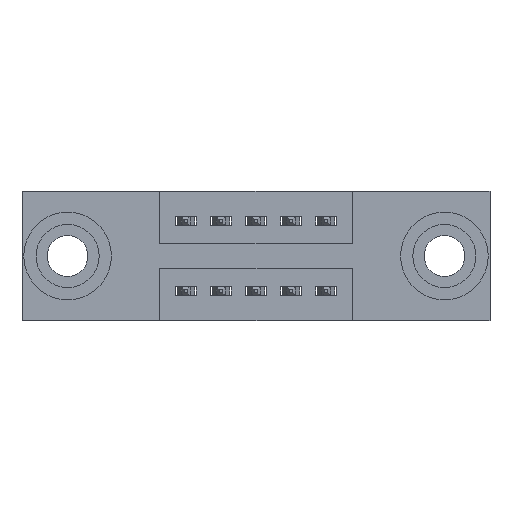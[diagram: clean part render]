
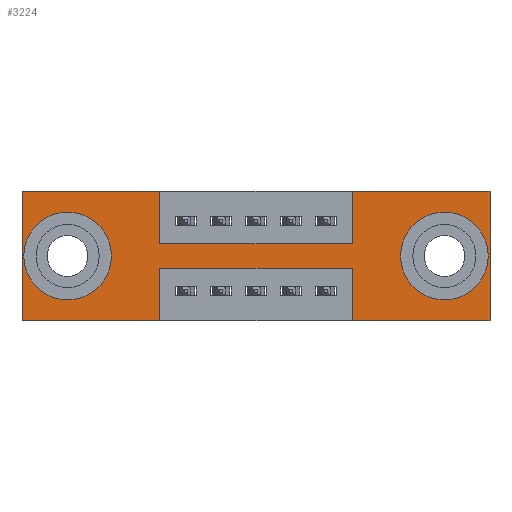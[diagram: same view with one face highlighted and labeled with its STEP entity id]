
A CAD part, front view. The second image highlights one B-rep face of the part: STEP entity #3224.
In plain terms, the highlighted planar face has unit normal (0, -1, 0).
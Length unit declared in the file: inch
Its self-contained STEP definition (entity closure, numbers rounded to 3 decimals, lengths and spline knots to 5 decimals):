
#199 = VERTEX_POINT ( 'NONE', #5408 ) ;
#202 = CARTESIAN_POINT ( 'NONE',  ( 0.9425, 0., -0.22 ) ) ;
#220 = VERTEX_POINT ( 'NONE', #5015 ) ;
#273 = LINE ( 'NONE', #3442, #8109 ) ;
#441 = CARTESIAN_POINT ( 'NONE',  ( 1.205, 0., -0.107 ) ) ;
#451 = EDGE_CURVE ( 'NONE', #7495, #7640, #5093, .T. ) ;
#491 = DIRECTION ( 'NONE',  ( 0., 1., 0. ) ) ;
#572 = AXIS2_PLACEMENT_3D ( 'NONE', #5320, #583, #6077 ) ;
#583 = DIRECTION ( 'NONE',  ( 0., 1., 0. ) ) ;
#598 = ORIENTED_EDGE ( 'NONE', *, *, #2854, .F. ) ;
#739 = VECTOR ( 'NONE', #2907, 39.37008 ) ;
#806 = EDGE_CURVE ( 'NONE', #3366, #220, #8985, .T. ) ;
#825 = VECTOR ( 'NONE', #2580, 39.37008 ) ;
#908 = VECTOR ( 'NONE', #1467, 39.37008 ) ;
#920 = EDGE_CURVE ( 'NONE', #6733, #3366, #6147, .T. ) ;
#1013 = ORIENTED_EDGE ( 'NONE', *, *, #6311, .F. ) ;
#1037 = VERTEX_POINT ( 'NONE', #5491 ) ;
#1129 = CARTESIAN_POINT ( 'NONE',  ( 0.9425, 0., 0. ) ) ;
#1196 = VERTEX_POINT ( 'NONE', #3708 ) ;
#1205 = VERTEX_POINT ( 'NONE', #3588 ) ;
#1379 = ORIENTED_EDGE ( 'NONE', *, *, #4823, .T. ) ;
#1417 = VECTOR ( 'NONE', #8301, 39.37008 ) ;
#1467 = DIRECTION ( 'NONE',  ( -1., 0., 0. ) ) ;
#1501 = FACE_OUTER_BOUND ( 'NONE', #8393, .T. ) ;
#1577 = CIRCLE ( 'NONE', #572, 0.078 ) ;
#1755 = CARTESIAN_POINT ( 'NONE',  ( 0., 0., 0. ) ) ;
#1802 = LINE ( 'NONE', #2672, #3683 ) ;
#1833 = DIRECTION ( 'NONE',  ( 0., 0., -1. ) ) ;
#1900 = ORIENTED_EDGE ( 'NONE', *, *, #8420, .F. ) ;
#1905 = CARTESIAN_POINT ( 'NONE',  ( 0.13, 0., -0.185 ) ) ;
#1915 = EDGE_LOOP ( 'NONE', ( #6055, #2595 ) ) ;
#2142 = DIRECTION ( 'NONE',  ( 0., 0., -1. ) ) ;
#2143 = DIRECTION ( 'NONE',  ( 0., 0., -1. ) ) ;
#2193 = DIRECTION ( 'NONE',  ( 0., 1., 0. ) ) ;
#2208 = CARTESIAN_POINT ( 'NONE',  ( 1.205, 0., -0.185 ) ) ;
#2414 = ORIENTED_EDGE ( 'NONE', *, *, #451, .F. ) ;
#2517 = CARTESIAN_POINT ( 'NONE',  ( 1.205, 0., -0.263 ) ) ;
#2550 = ORIENTED_EDGE ( 'NONE', *, *, #7188, .F. ) ;
#2556 = VECTOR ( 'NONE', #6712, 39.37008 ) ;
#2576 = CARTESIAN_POINT ( 'NONE',  ( 0.9425, 0., -0.37 ) ) ;
#2580 = DIRECTION ( 'NONE',  ( 0., 0., 1. ) ) ;
#2595 = ORIENTED_EDGE ( 'NONE', *, *, #6934, .T. ) ;
#2665 = ORIENTED_EDGE ( 'NONE', *, *, #6577, .F. ) ;
#2672 = CARTESIAN_POINT ( 'NONE',  ( 0.3925, 0., -0.22 ) ) ;
#2674 = ORIENTED_EDGE ( 'NONE', *, *, #806, .F. ) ;
#2739 = DIRECTION ( 'NONE',  ( 0., 0., 1. ) ) ;
#2854 = EDGE_CURVE ( 'NONE', #1037, #7495, #6874, .T. ) ;
#2907 = DIRECTION ( 'NONE',  ( 0., 0., -1. ) ) ;
#2994 = LINE ( 'NONE', #2576, #825 ) ;
#3038 = CARTESIAN_POINT ( 'NONE',  ( 1.335, 0., 0. ) ) ;
#3046 = PLANE ( 'NONE',  #9576 ) ;
#3081 = ORIENTED_EDGE ( 'NONE', *, *, #9064, .F. ) ;
#3224 = ADVANCED_FACE ( 'NONE', ( #3406, #5167, #1501 ), #3046, .T. ) ;
#3263 = DIRECTION ( 'NONE',  ( 1., 0., 0. ) ) ;
#3272 = CARTESIAN_POINT ( 'NONE',  ( 0.3925, 0., -0.22 ) ) ;
#3359 = LINE ( 'NONE', #4021, #8809 ) ;
#3366 = VERTEX_POINT ( 'NONE', #1755 ) ;
#3406 = FACE_BOUND ( 'NONE', #7804, .T. ) ;
#3442 = CARTESIAN_POINT ( 'NONE',  ( 0.3925, 0., 0. ) ) ;
#3456 = LINE ( 'NONE', #1129, #5235 ) ;
#3463 = LINE ( 'NONE', #7214, #7792 ) ;
#3573 = LINE ( 'NONE', #5459, #9006 ) ;
#3574 = CARTESIAN_POINT ( 'NONE',  ( 0.13, 0., -0.107 ) ) ;
#3588 = CARTESIAN_POINT ( 'NONE',  ( 0.3925, 0., -0.15 ) ) ;
#3683 = VECTOR ( 'NONE', #9095, 39.37008 ) ;
#3703 = VERTEX_POINT ( 'NONE', #6183 ) ;
#3708 = CARTESIAN_POINT ( 'NONE',  ( 0.9425, 0., 0. ) ) ;
#3726 = DIRECTION ( 'NONE',  ( 0., -1., 0. ) ) ;
#3761 = CARTESIAN_POINT ( 'NONE',  ( 0., 0., -0.37 ) ) ;
#4021 = CARTESIAN_POINT ( 'NONE',  ( 0.3925, 0., -0.15 ) ) ;
#4080 = CIRCLE ( 'NONE', #7182, 0.078 ) ;
#4277 = DIRECTION ( 'NONE',  ( 0., 0., 1. ) ) ;
#4473 = ORIENTED_EDGE ( 'NONE', *, *, #5335, .F. ) ;
#4524 = VERTEX_POINT ( 'NONE', #3272 ) ;
#4554 = ORIENTED_EDGE ( 'NONE', *, *, #8476, .F. ) ;
#4625 = CARTESIAN_POINT ( 'NONE',  ( 1.335, 0., -0.37 ) ) ;
#4750 = CIRCLE ( 'NONE', #5298, 0.078 ) ;
#4823 = EDGE_CURVE ( 'NONE', #5206, #9169, #4080, .T. ) ;
#5015 = CARTESIAN_POINT ( 'NONE',  ( 0.3925, 0., 0. ) ) ;
#5070 = DIRECTION ( 'NONE',  ( 0., 0., -1. ) ) ;
#5093 = LINE ( 'NONE', #5164, #908 ) ;
#5164 = CARTESIAN_POINT ( 'NONE',  ( 0., 0., -0.37 ) ) ;
#5167 = FACE_BOUND ( 'NONE', #1915, .T. ) ;
#5206 = VERTEX_POINT ( 'NONE', #441 ) ;
#5231 = ORIENTED_EDGE ( 'NONE', *, *, #7355, .F. ) ;
#5235 = VECTOR ( 'NONE', #4277, 39.37008 ) ;
#5251 = CARTESIAN_POINT ( 'NONE',  ( 1.205, 0., -0.185 ) ) ;
#5298 = AXIS2_PLACEMENT_3D ( 'NONE', #5251, #491, #5998 ) ;
#5320 = CARTESIAN_POINT ( 'NONE',  ( 0.13, 0., -0.185 ) ) ;
#5335 = EDGE_CURVE ( 'NONE', #7640, #5436, #2994, .T. ) ;
#5408 = CARTESIAN_POINT ( 'NONE',  ( 0.9425, 0., -0.15 ) ) ;
#5436 = VERTEX_POINT ( 'NONE', #202 ) ;
#5459 = CARTESIAN_POINT ( 'NONE',  ( 0., 0., -0.37 ) ) ;
#5491 = CARTESIAN_POINT ( 'NONE',  ( 1.335, 0., 0. ) ) ;
#5998 = DIRECTION ( 'NONE',  ( 0., 0., -1. ) ) ;
#6055 = ORIENTED_EDGE ( 'NONE', *, *, #6650, .T. ) ;
#6077 = DIRECTION ( 'NONE',  ( 0., 0., 1. ) ) ;
#6106 = ORIENTED_EDGE ( 'NONE', *, *, #9574, .T. ) ;
#6147 = LINE ( 'NONE', #6682, #2556 ) ;
#6183 = CARTESIAN_POINT ( 'NONE',  ( 0.3925, 0., -0.37 ) ) ;
#6311 = EDGE_CURVE ( 'NONE', #3703, #6733, #3573, .T. ) ;
#6344 = VERTEX_POINT ( 'NONE', #9570 ) ;
#6471 = VECTOR ( 'NONE', #8275, 39.37008 ) ;
#6541 = ORIENTED_EDGE ( 'NONE', *, *, #920, .F. ) ;
#6577 = EDGE_CURVE ( 'NONE', #220, #1205, #273, .T. ) ;
#6650 = EDGE_CURVE ( 'NONE', #7959, #6344, #7898, .T. ) ;
#6682 = CARTESIAN_POINT ( 'NONE',  ( 0., 0., 0. ) ) ;
#6712 = DIRECTION ( 'NONE',  ( 0., 0., 1. ) ) ;
#6733 = VERTEX_POINT ( 'NONE', #7963 ) ;
#6874 = LINE ( 'NONE', #3038, #739 ) ;
#6934 = EDGE_CURVE ( 'NONE', #6344, #7959, #1577, .T. ) ;
#7182 = AXIS2_PLACEMENT_3D ( 'NONE', #2208, #2193, #2143 ) ;
#7188 = EDGE_CURVE ( 'NONE', #1205, #199, #3359, .T. ) ;
#7192 = DIRECTION ( 'NONE',  ( 0., 1., 0. ) ) ;
#7214 = CARTESIAN_POINT ( 'NONE',  ( 0.3925, 0., -0.37 ) ) ;
#7355 = EDGE_CURVE ( 'NONE', #4524, #3703, #3463, .T. ) ;
#7436 = AXIS2_PLACEMENT_3D ( 'NONE', #1905, #7192, #2739 ) ;
#7495 = VERTEX_POINT ( 'NONE', #4625 ) ;
#7621 = CARTESIAN_POINT ( 'NONE',  ( 0., 0., 0. ) ) ;
#7640 = VERTEX_POINT ( 'NONE', #9552 ) ;
#7792 = VECTOR ( 'NONE', #5070, 39.37008 ) ;
#7804 = EDGE_LOOP ( 'NONE', ( #1379, #6106 ) ) ;
#7898 = CIRCLE ( 'NONE', #7436, 0.078 ) ;
#7959 = VERTEX_POINT ( 'NONE', #3574 ) ;
#7963 = CARTESIAN_POINT ( 'NONE',  ( 0., 0., -0.37 ) ) ;
#8109 = VECTOR ( 'NONE', #1833, 39.37008 ) ;
#8236 = CARTESIAN_POINT ( 'NONE',  ( 0., 0., 0. ) ) ;
#8275 = DIRECTION ( 'NONE',  ( 1., 0., 0. ) ) ;
#8282 = LINE ( 'NONE', #7621, #6471 ) ;
#8301 = DIRECTION ( 'NONE',  ( 1., 0., 0. ) ) ;
#8393 = EDGE_LOOP ( 'NONE', ( #5231, #1900, #4473, #2414, #598, #3081, #4554, #2550, #2665, #2674, #6541, #1013 ) ) ;
#8420 = EDGE_CURVE ( 'NONE', #5436, #4524, #1802, .T. ) ;
#8476 = EDGE_CURVE ( 'NONE', #199, #1196, #3456, .T. ) ;
#8809 = VECTOR ( 'NONE', #3263, 39.37008 ) ;
#8985 = LINE ( 'NONE', #8236, #1417 ) ;
#9006 = VECTOR ( 'NONE', #9545, 39.37008 ) ;
#9064 = EDGE_CURVE ( 'NONE', #1196, #1037, #8282, .T. ) ;
#9095 = DIRECTION ( 'NONE',  ( -1., 0., 0. ) ) ;
#9169 = VERTEX_POINT ( 'NONE', #2517 ) ;
#9545 = DIRECTION ( 'NONE',  ( -1., 0., 0. ) ) ;
#9552 = CARTESIAN_POINT ( 'NONE',  ( 0.9425, 0., -0.37 ) ) ;
#9570 = CARTESIAN_POINT ( 'NONE',  ( 0.13, 0., -0.263 ) ) ;
#9574 = EDGE_CURVE ( 'NONE', #9169, #5206, #4750, .T. ) ;
#9576 = AXIS2_PLACEMENT_3D ( 'NONE', #3761, #3726, #2142 ) ;
